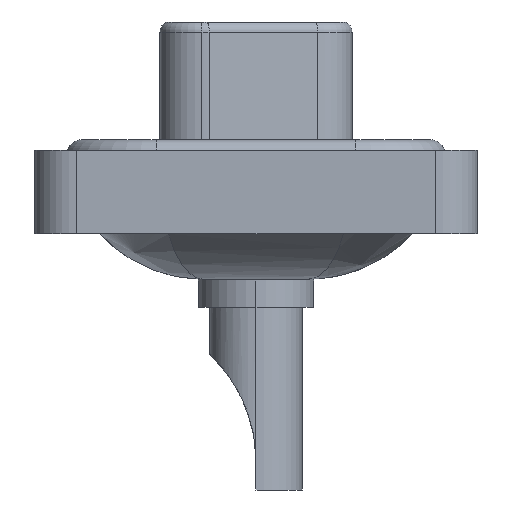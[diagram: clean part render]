
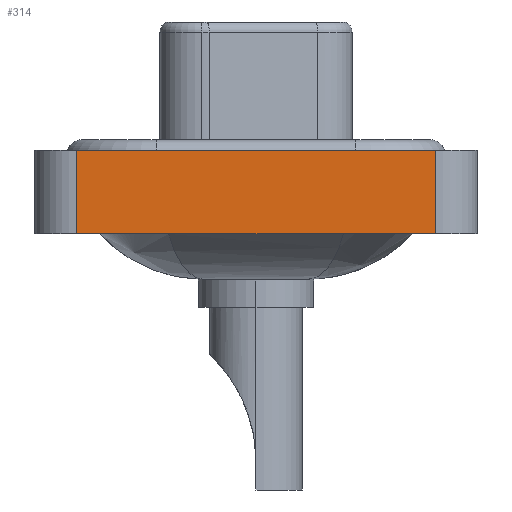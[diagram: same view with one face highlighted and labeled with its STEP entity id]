
A CAD part, left-side view. The second image highlights one B-rep face of the part: STEP entity #314.
In plain terms, the highlighted planar face has unit normal (-1, 0, 0).
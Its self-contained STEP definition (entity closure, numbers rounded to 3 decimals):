
#314 = ADVANCED_FACE ( 'NONE', ( #19463 ), #5707, .T. ) ;
#476 = CARTESIAN_POINT ( 'NONE',  ( -7.3, -8.55, -3.6 ) ) ;
#486 = EDGE_CURVE ( 'NONE', #18298, #16617, #3972, .T. ) ;
#597 = ORIENTED_EDGE ( 'NONE', *, *, #16156, .F. ) ;
#1620 = EDGE_CURVE ( 'NONE', #18298, #11831, #14240, .T. ) ;
#3261 = CARTESIAN_POINT ( 'NONE',  ( -7.3, -8.55, 0.4 ) ) ;
#3972 = LINE ( 'NONE', #16234, #7714 ) ;
#4198 = DIRECTION ( 'NONE',  ( -1., 0., 0. ) ) ;
#4393 = CARTESIAN_POINT ( 'NONE',  ( -7.3, -8.55, -3.6 ) ) ;
#4522 = ORIENTED_EDGE ( 'NONE', *, *, #486, .F. ) ;
#4575 = CARTESIAN_POINT ( 'NONE',  ( -7.3, 8.55, 0.4 ) ) ;
#4885 = LINE ( 'NONE', #9514, #13969 ) ;
#5035 = CARTESIAN_POINT ( 'NONE',  ( -7.3, -8.55, -3.6 ) ) ;
#5088 = DIRECTION ( 'NONE',  ( 0., -1., 0. ) ) ;
#5495 = EDGE_LOOP ( 'NONE', ( #9587, #597, #4522, #5764 ) ) ;
#5707 = PLANE ( 'NONE',  #13477 ) ;
#5764 = ORIENTED_EDGE ( 'NONE', *, *, #1620, .T. ) ;
#5873 = CARTESIAN_POINT ( 'NONE',  ( -7.3, -8.55, -3.6 ) ) ;
#6451 = VERTEX_POINT ( 'NONE', #3261 ) ;
#6652 = DIRECTION ( 'NONE',  ( 0., 0., 1. ) ) ;
#7384 = CARTESIAN_POINT ( 'NONE',  ( -7.3, 8.55, -3.6 ) ) ;
#7714 = VECTOR ( 'NONE', #17935, 1000. ) ;
#9514 = CARTESIAN_POINT ( 'NONE',  ( -7.3, -8.55, 0.4 ) ) ;
#9587 = ORIENTED_EDGE ( 'NONE', *, *, #14185, .T. ) ;
#10911 = DIRECTION ( 'NONE',  ( 0., -1., 0. ) ) ;
#11831 = VERTEX_POINT ( 'NONE', #5873 ) ;
#13477 = AXIS2_PLACEMENT_3D ( 'NONE', #4393, #4198, #16647 ) ;
#13678 = VECTOR ( 'NONE', #6652, 1000. ) ;
#13969 = VECTOR ( 'NONE', #5088, 1000. ) ;
#14178 = VECTOR ( 'NONE', #10911, 1000. ) ;
#14185 = EDGE_CURVE ( 'NONE', #11831, #6451, #17305, .T. ) ;
#14240 = LINE ( 'NONE', #476, #14178 ) ;
#16156 = EDGE_CURVE ( 'NONE', #16617, #6451, #4885, .T. ) ;
#16234 = CARTESIAN_POINT ( 'NONE',  ( -7.3, 8.55, -3.6 ) ) ;
#16617 = VERTEX_POINT ( 'NONE', #4575 ) ;
#16647 = DIRECTION ( 'NONE',  ( 0., 0., 1. ) ) ;
#17305 = LINE ( 'NONE', #5035, #13678 ) ;
#17935 = DIRECTION ( 'NONE',  ( 0., 0., 1. ) ) ;
#18298 = VERTEX_POINT ( 'NONE', #7384 ) ;
#19463 = FACE_OUTER_BOUND ( 'NONE', #5495, .T. ) ;
